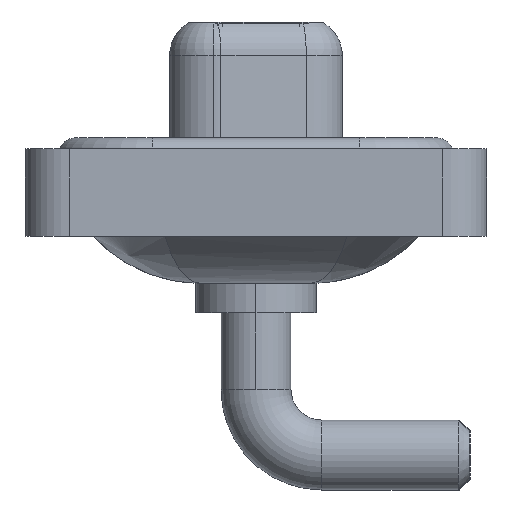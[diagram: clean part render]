
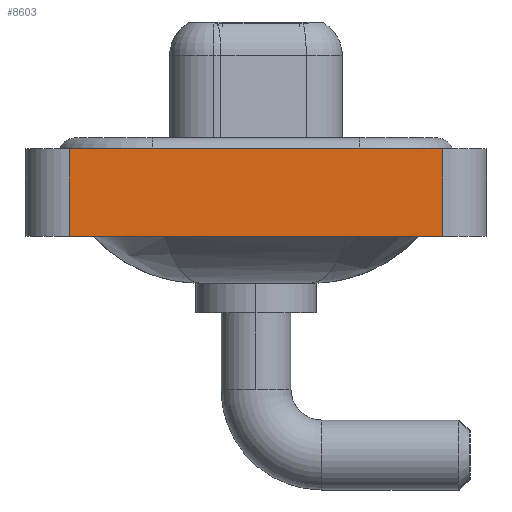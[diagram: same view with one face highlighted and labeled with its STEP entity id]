
A CAD part, left-side view. The second image highlights one B-rep face of the part: STEP entity #8603.
In plain terms, the highlighted planar face has unit normal (-1, 0, 0).
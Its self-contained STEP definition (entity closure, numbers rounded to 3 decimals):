
#179 = VECTOR ( 'NONE', #14246, 1000. ) ;
#301 = CARTESIAN_POINT ( 'NONE',  ( -7.3, 8.55, 0.4 ) ) ;
#1228 = ORIENTED_EDGE ( 'NONE', *, *, #1492, .T. ) ;
#1306 = DIRECTION ( 'NONE',  ( 0., 0., 1. ) ) ;
#1492 = EDGE_CURVE ( 'NONE', #3220, #9316, #4073, .T. ) ;
#1865 = VERTEX_POINT ( 'NONE', #14638 ) ;
#2682 = DIRECTION ( 'NONE',  ( 0., -1., 0. ) ) ;
#2695 = VERTEX_POINT ( 'NONE', #301 ) ;
#3062 = DIRECTION ( 'NONE',  ( 0., 0., 1. ) ) ;
#3220 = VERTEX_POINT ( 'NONE', #9328 ) ;
#3971 = PLANE ( 'NONE',  #13445 ) ;
#4073 = LINE ( 'NONE', #7929, #7917 ) ;
#5314 = VECTOR ( 'NONE', #3062, 1000. ) ;
#7080 = ORIENTED_EDGE ( 'NONE', *, *, #11069, .F. ) ;
#7917 = VECTOR ( 'NONE', #13271, 1000. ) ;
#7929 = CARTESIAN_POINT ( 'NONE',  ( -7.3, -8.55, -3.6 ) ) ;
#7993 = FACE_OUTER_BOUND ( 'NONE', #11868, .T. ) ;
#8603 = ADVANCED_FACE ( 'NONE', ( #7993 ), #3971, .T. ) ;
#9316 = VERTEX_POINT ( 'NONE', #15353 ) ;
#9328 = CARTESIAN_POINT ( 'NONE',  ( -7.3, -8.55, -3.6 ) ) ;
#10091 = ORIENTED_EDGE ( 'NONE', *, *, #13547, .T. ) ;
#10594 = ORIENTED_EDGE ( 'NONE', *, *, #16280, .F. ) ;
#11069 = EDGE_CURVE ( 'NONE', #1865, #2695, #13748, .T. ) ;
#11868 = EDGE_LOOP ( 'NONE', ( #1228, #10594, #7080, #10091 ) ) ;
#12421 = CARTESIAN_POINT ( 'NONE',  ( -7.3, -8.55, 0.4 ) ) ;
#13176 = CARTESIAN_POINT ( 'NONE',  ( -7.3, -8.55, -3.6 ) ) ;
#13271 = DIRECTION ( 'NONE',  ( 0., 0., 1. ) ) ;
#13445 = AXIS2_PLACEMENT_3D ( 'NONE', #13176, #14487, #1306 ) ;
#13547 = EDGE_CURVE ( 'NONE', #1865, #3220, #16971, .T. ) ;
#13748 = LINE ( 'NONE', #15335, #5314 ) ;
#14173 = VECTOR ( 'NONE', #2682, 1000. ) ;
#14246 = DIRECTION ( 'NONE',  ( 0., -1., 0. ) ) ;
#14487 = DIRECTION ( 'NONE',  ( -1., 0., 0. ) ) ;
#14638 = CARTESIAN_POINT ( 'NONE',  ( -7.3, 8.55, -3.6 ) ) ;
#14876 = LINE ( 'NONE', #12421, #14173 ) ;
#15335 = CARTESIAN_POINT ( 'NONE',  ( -7.3, 8.55, -3.6 ) ) ;
#15353 = CARTESIAN_POINT ( 'NONE',  ( -7.3, -8.55, 0.4 ) ) ;
#15653 = CARTESIAN_POINT ( 'NONE',  ( -7.3, -8.55, -3.6 ) ) ;
#16280 = EDGE_CURVE ( 'NONE', #2695, #9316, #14876, .T. ) ;
#16971 = LINE ( 'NONE', #15653, #179 ) ;
